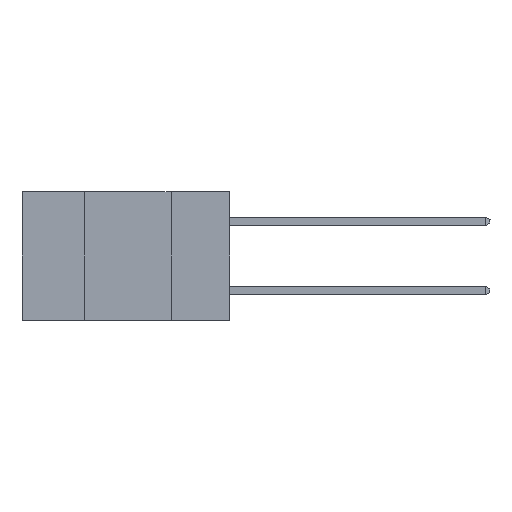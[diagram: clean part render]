
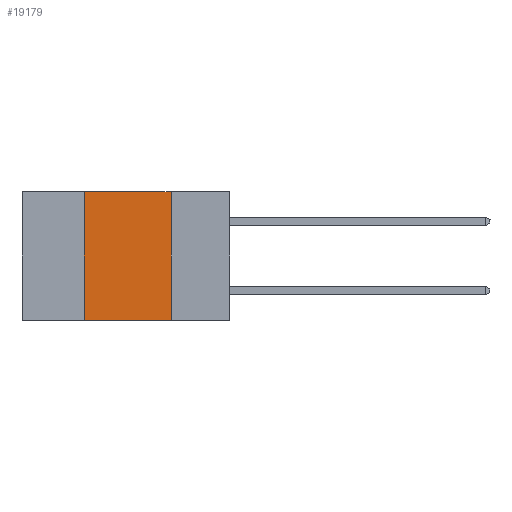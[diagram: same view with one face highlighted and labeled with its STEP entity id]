
A CAD part, left-side view. The second image highlights one B-rep face of the part: STEP entity #19179.
In plain terms, the highlighted planar face has unit normal (-1, 0, 0).
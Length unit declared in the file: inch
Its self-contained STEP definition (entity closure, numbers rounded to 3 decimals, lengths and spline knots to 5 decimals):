
#422 = CARTESIAN_POINT ( 'NONE',  ( 0., 0.42, 0. ) ) ;
#846 = ORIENTED_EDGE ( 'NONE', *, *, #19617, .F. ) ;
#899 = LINE ( 'NONE', #4851, #10180 ) ;
#1348 = VECTOR ( 'NONE', #12183, 39.37008 ) ;
#1495 = DIRECTION ( 'NONE',  ( 1., 0., 0. ) ) ;
#2539 = DIRECTION ( 'NONE',  ( 0., -1., 0. ) ) ;
#3059 = ORIENTED_EDGE ( 'NONE', *, *, #14558, .F. ) ;
#3422 = ORIENTED_EDGE ( 'NONE', *, *, #10207, .T. ) ;
#3883 = CARTESIAN_POINT ( 'NONE',  ( 0., 0.17, 0. ) ) ;
#3938 = LINE ( 'NONE', #14756, #12099 ) ;
#4851 = CARTESIAN_POINT ( 'NONE',  ( 0., 0.6, -0.37 ) ) ;
#6629 = DIRECTION ( 'NONE',  ( 0., -1., 0. ) ) ;
#8099 = ORIENTED_EDGE ( 'NONE', *, *, #12369, .F. ) ;
#8459 = PLANE ( 'NONE',  #9398 ) ;
#9056 = DIRECTION ( 'NONE',  ( 0., 0., -1. ) ) ;
#9398 = AXIS2_PLACEMENT_3D ( 'NONE', #10037, #1495, #13682 ) ;
#10037 = CARTESIAN_POINT ( 'NONE',  ( 0., 0.6, 0. ) ) ;
#10180 = VECTOR ( 'NONE', #6629, 39.37008 ) ;
#10207 = EDGE_CURVE ( 'NONE', #11782, #11662, #899, .T. ) ;
#10455 = CARTESIAN_POINT ( 'NONE',  ( 0., 0.17, -0.37 ) ) ;
#10624 = LINE ( 'NONE', #422, #1348 ) ;
#10676 = CARTESIAN_POINT ( 'NONE',  ( 0., 0.42, -0.37 ) ) ;
#11662 = VERTEX_POINT ( 'NONE', #10455 ) ;
#11782 = VERTEX_POINT ( 'NONE', #10676 ) ;
#12099 = VECTOR ( 'NONE', #2539, 39.37008 ) ;
#12183 = DIRECTION ( 'NONE',  ( 0., 0., 1. ) ) ;
#12369 = EDGE_CURVE ( 'NONE', #11782, #13008, #10624, .T. ) ;
#12715 = LINE ( 'NONE', #3883, #13257 ) ;
#13008 = VERTEX_POINT ( 'NONE', #14301 ) ;
#13257 = VECTOR ( 'NONE', #9056, 39.37008 ) ;
#13682 = DIRECTION ( 'NONE',  ( 0., 0., -1. ) ) ;
#14301 = CARTESIAN_POINT ( 'NONE',  ( 0., 0.42, 0. ) ) ;
#14558 = EDGE_CURVE ( 'NONE', #16709, #11662, #12715, .T. ) ;
#14756 = CARTESIAN_POINT ( 'NONE',  ( 0., 0.6, 0. ) ) ;
#16709 = VERTEX_POINT ( 'NONE', #16815 ) ;
#16815 = CARTESIAN_POINT ( 'NONE',  ( 0., 0.17, 0. ) ) ;
#17215 = FACE_OUTER_BOUND ( 'NONE', #21182, .T. ) ;
#19179 = ADVANCED_FACE ( 'NONE', ( #17215 ), #8459, .F. ) ;
#19617 = EDGE_CURVE ( 'NONE', #13008, #16709, #3938, .T. ) ;
#21182 = EDGE_LOOP ( 'NONE', ( #3059, #846, #8099, #3422 ) ) ;
